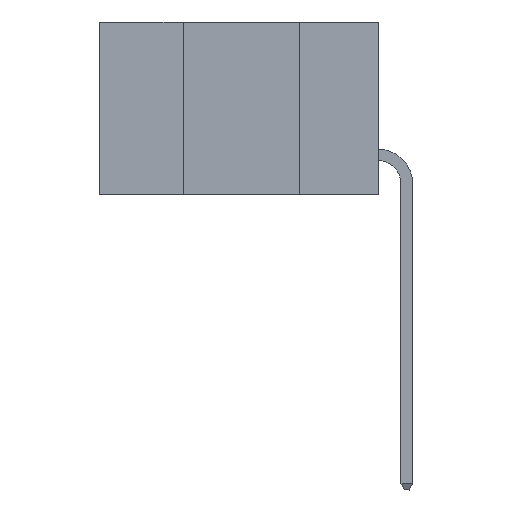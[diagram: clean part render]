
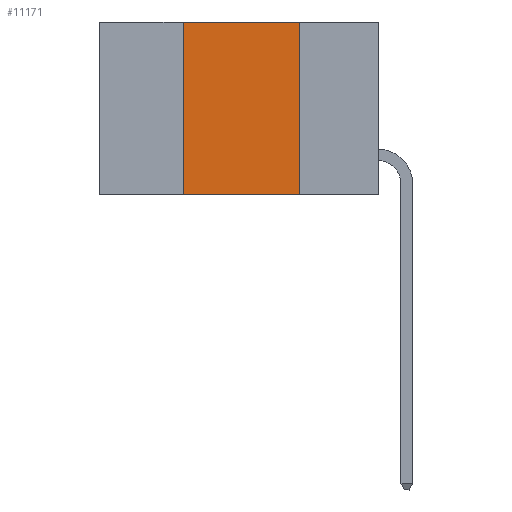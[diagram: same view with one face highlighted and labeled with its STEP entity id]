
A CAD part, left-side view. The second image highlights one B-rep face of the part: STEP entity #11171.
In plain terms, the highlighted planar face has unit normal (-1, 0, 0).
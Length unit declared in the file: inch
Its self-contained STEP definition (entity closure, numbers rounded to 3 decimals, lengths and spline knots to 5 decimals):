
#1293 = VECTOR ( 'NONE', #16223, 39.37008 ) ;
#1487 = VECTOR ( 'NONE', #4355, 39.37008 ) ;
#2219 = CARTESIAN_POINT ( 'NONE',  ( 0., 0.42, 0. ) ) ;
#2238 = FACE_OUTER_BOUND ( 'NONE', #23556, .T. ) ;
#2889 = DIRECTION ( 'NONE',  ( 0., -1., 0. ) ) ;
#3080 = LINE ( 'NONE', #2219, #1487 ) ;
#4014 = CARTESIAN_POINT ( 'NONE',  ( 0., 0.17, -0.37 ) ) ;
#4355 = DIRECTION ( 'NONE',  ( 0., 0., 1. ) ) ;
#4375 = DIRECTION ( 'NONE',  ( 0., 0., -1. ) ) ;
#5130 = CARTESIAN_POINT ( 'NONE',  ( 0., 0.6, -0.37 ) ) ;
#5436 = DIRECTION ( 'NONE',  ( 1., 0., 0. ) ) ;
#5890 = ORIENTED_EDGE ( 'NONE', *, *, #23251, .F. ) ;
#6094 = CARTESIAN_POINT ( 'NONE',  ( 0., 0.17, 0. ) ) ;
#6310 = ORIENTED_EDGE ( 'NONE', *, *, #8689, .F. ) ;
#6724 = CARTESIAN_POINT ( 'NONE',  ( 0., 0.17, 0. ) ) ;
#6947 = VERTEX_POINT ( 'NONE', #13403 ) ;
#7782 = VECTOR ( 'NONE', #4375, 39.37008 ) ;
#7991 = VERTEX_POINT ( 'NONE', #4014 ) ;
#8689 = EDGE_CURVE ( 'NONE', #6947, #18640, #26301, .T. ) ;
#9723 = DIRECTION ( 'NONE',  ( 0., 0., -1. ) ) ;
#11171 = ADVANCED_FACE ( 'NONE', ( #2238 ), #11676, .F. ) ;
#11676 = PLANE ( 'NONE',  #14260 ) ;
#13403 = CARTESIAN_POINT ( 'NONE',  ( 0., 0.42, 0. ) ) ;
#13890 = LINE ( 'NONE', #6094, #7782 ) ;
#14260 = AXIS2_PLACEMENT_3D ( 'NONE', #15802, #5436, #9723 ) ;
#15802 = CARTESIAN_POINT ( 'NONE',  ( 0., 0.6, 0. ) ) ;
#15973 = LINE ( 'NONE', #5130, #16940 ) ;
#16223 = DIRECTION ( 'NONE',  ( 0., -1., 0. ) ) ;
#16940 = VECTOR ( 'NONE', #2889, 39.37008 ) ;
#17967 = EDGE_CURVE ( 'NONE', #23098, #7991, #15973, .T. ) ;
#18640 = VERTEX_POINT ( 'NONE', #6724 ) ;
#20010 = EDGE_CURVE ( 'NONE', #23098, #6947, #3080, .T. ) ;
#20155 = CARTESIAN_POINT ( 'NONE',  ( 0., 0.6, 0. ) ) ;
#23098 = VERTEX_POINT ( 'NONE', #26130 ) ;
#23251 = EDGE_CURVE ( 'NONE', #18640, #7991, #13890, .T. ) ;
#23556 = EDGE_LOOP ( 'NONE', ( #5890, #6310, #25127, #23705 ) ) ;
#23705 = ORIENTED_EDGE ( 'NONE', *, *, #17967, .T. ) ;
#25127 = ORIENTED_EDGE ( 'NONE', *, *, #20010, .F. ) ;
#26130 = CARTESIAN_POINT ( 'NONE',  ( 0., 0.42, -0.37 ) ) ;
#26301 = LINE ( 'NONE', #20155, #1293 ) ;
